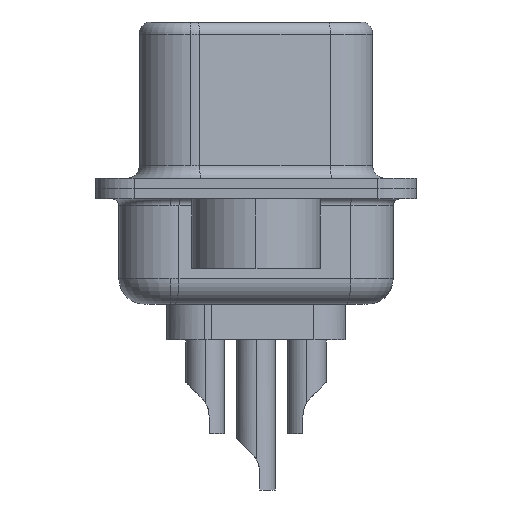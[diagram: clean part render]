
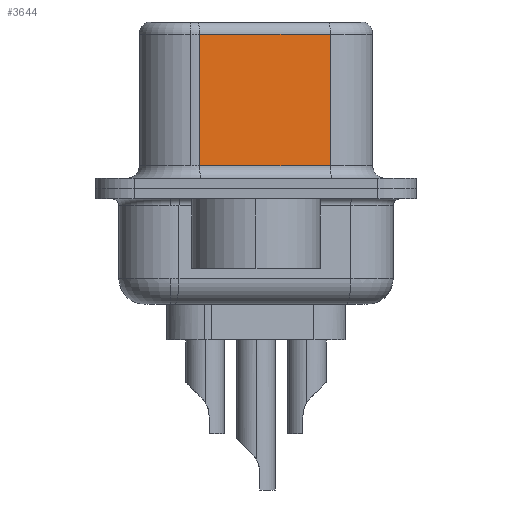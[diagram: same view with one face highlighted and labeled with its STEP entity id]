
A CAD part, left-side view. The second image highlights one B-rep face of the part: STEP entity #3644.
In plain terms, the highlighted planar face has unit normal (-0.985, -0.174, 0).
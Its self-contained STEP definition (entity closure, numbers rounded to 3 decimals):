
#379 = VERTEX_POINT ( 'NONE', #12684 ) ;
#685 = AXIS2_PLACEMENT_3D ( 'NONE', #4845, #12618, #2229 ) ;
#1509 = VERTEX_POINT ( 'NONE', #17130 ) ;
#1597 = VERTEX_POINT ( 'NONE', #11231 ) ;
#1949 = ORIENTED_EDGE ( 'NONE', *, *, #5136, .T. ) ;
#2229 = DIRECTION ( 'NONE',  ( -0.174, 0.985, 0. ) ) ;
#2472 = ORIENTED_EDGE ( 'NONE', *, *, #14279, .T. ) ;
#2808 = EDGE_LOOP ( 'NONE', ( #9498, #2472, #1949, #6275 ) ) ;
#3644 = ADVANCED_FACE ( 'NONE', ( #14581 ), #10633, .F. ) ;
#4147 = CARTESIAN_POINT ( 'NONE',  ( 3.655, 2.203, 6.52 ) ) ;
#4404 = DIRECTION ( 'NONE',  ( -0.174, 0.985, 0. ) ) ;
#4736 = VECTOR ( 'NONE', #7518, 1000. ) ;
#4845 = CARTESIAN_POINT ( 'NONE',  ( 4.555, -2.897, 6.52 ) ) ;
#5136 = EDGE_CURVE ( 'NONE', #12475, #379, #9086, .T. ) ;
#5684 = DIRECTION ( 'NONE',  ( 0.174, -0.985, 0. ) ) ;
#6275 = ORIENTED_EDGE ( 'NONE', *, *, #6866, .T. ) ;
#6866 = EDGE_CURVE ( 'NONE', #379, #1509, #20530, .T. ) ;
#7383 = VECTOR ( 'NONE', #4404, 1000. ) ;
#7518 = DIRECTION ( 'NONE',  ( 0., 0., -1. ) ) ;
#8984 = DIRECTION ( 'NONE',  ( 0., 0., -1. ) ) ;
#9086 = LINE ( 'NONE', #4147, #4736 ) ;
#9304 = VECTOR ( 'NONE', #8984, 1000. ) ;
#9498 = ORIENTED_EDGE ( 'NONE', *, *, #10092, .F. ) ;
#10092 = EDGE_CURVE ( 'NONE', #1597, #1509, #17183, .T. ) ;
#10633 = PLANE ( 'NONE',  #685 ) ;
#10899 = CARTESIAN_POINT ( 'NONE',  ( 4.555, -2.897, 0.9 ) ) ;
#11231 = CARTESIAN_POINT ( 'NONE',  ( 4.555, -2.897, 6.02 ) ) ;
#12475 = VERTEX_POINT ( 'NONE', #19609 ) ;
#12618 = DIRECTION ( 'NONE',  ( 0.985, 0.174, 0. ) ) ;
#12684 = CARTESIAN_POINT ( 'NONE',  ( 3.655, 2.203, 0.9 ) ) ;
#14048 = CARTESIAN_POINT ( 'NONE',  ( 4.555, -2.897, 6.02 ) ) ;
#14279 = EDGE_CURVE ( 'NONE', #1597, #12475, #15812, .T. ) ;
#14581 = FACE_OUTER_BOUND ( 'NONE', #2808, .T. ) ;
#15812 = LINE ( 'NONE', #14048, #7383 ) ;
#16436 = VECTOR ( 'NONE', #5684, 1000. ) ;
#17130 = CARTESIAN_POINT ( 'NONE',  ( 4.555, -2.897, 0.9 ) ) ;
#17183 = LINE ( 'NONE', #18388, #9304 ) ;
#18388 = CARTESIAN_POINT ( 'NONE',  ( 4.555, -2.897, 6.52 ) ) ;
#19609 = CARTESIAN_POINT ( 'NONE',  ( 3.655, 2.203, 6.02 ) ) ;
#20530 = LINE ( 'NONE', #10899, #16436 ) ;
